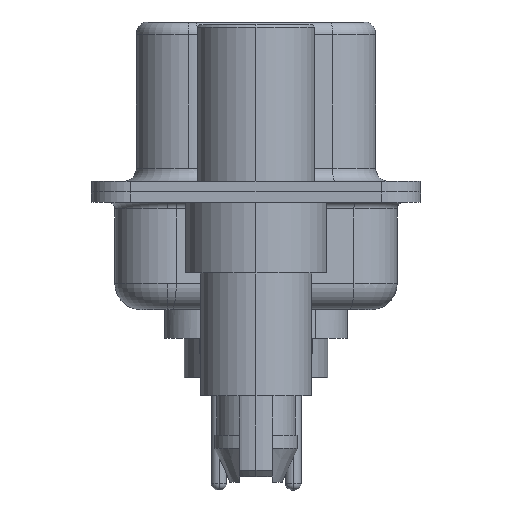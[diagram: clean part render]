
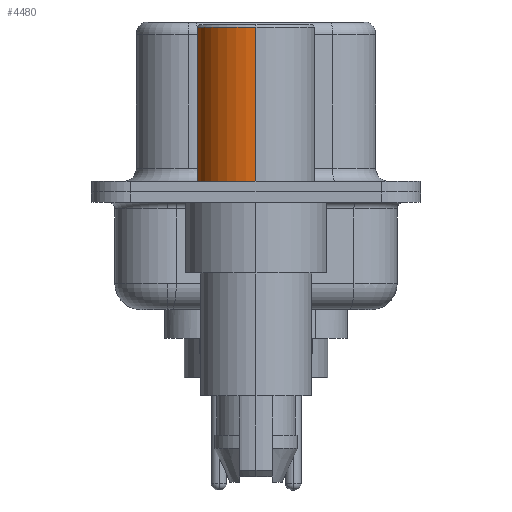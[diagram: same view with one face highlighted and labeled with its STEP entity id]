
A CAD part, left-side view. The second image highlights one B-rep face of the part: STEP entity #4480.
In plain terms, the highlighted cylindrical face has radius 2.25 mm (diameter 4.5 mm), a partial arc.
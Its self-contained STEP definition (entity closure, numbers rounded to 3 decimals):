
#163 = CIRCLE ( 'NONE', #2171, 2.25 ) ;
#1712 = CYLINDRICAL_SURFACE ( 'NONE', #19485, 2.25 ) ;
#1921 = CARTESIAN_POINT ( 'NONE',  ( 0., 0., 6.3 ) ) ;
#2171 = AXIS2_PLACEMENT_3D ( 'NONE', #12590, #12512, #12426 ) ;
#2316 = LINE ( 'NONE', #9059, #10362 ) ;
#3195 = CIRCLE ( 'NONE', #5423, 2.25 ) ;
#3201 = VERTEX_POINT ( 'NONE', #20568 ) ;
#3475 = ORIENTED_EDGE ( 'NONE', *, *, #18322, .F. ) ;
#3570 = DIRECTION ( 'NONE',  ( 1., 0., 0. ) ) ;
#3793 = EDGE_CURVE ( 'NONE', #5010, #3201, #163, .T. ) ;
#4480 = ADVANCED_FACE ( 'NONE', ( #14508 ), #1712, .T. ) ;
#5010 = VERTEX_POINT ( 'NONE', #9778 ) ;
#5423 = AXIS2_PLACEMENT_3D ( 'NONE', #1921, #13178, #3570 ) ;
#6766 = DIRECTION ( 'NONE',  ( 0., 0., 1. ) ) ;
#7247 = ORIENTED_EDGE ( 'NONE', *, *, #20223, .F. ) ;
#8501 = EDGE_CURVE ( 'NONE', #3201, #12145, #2316, .T. ) ;
#8787 = ORIENTED_EDGE ( 'NONE', *, *, #8501, .T. ) ;
#8957 = CARTESIAN_POINT ( 'NONE',  ( -2.25, 0., 6.3 ) ) ;
#9059 = CARTESIAN_POINT ( 'NONE',  ( -2.25, 0., 0.581 ) ) ;
#9778 = CARTESIAN_POINT ( 'NONE',  ( 2.25, 0., 0.4 ) ) ;
#9941 = CARTESIAN_POINT ( 'NONE',  ( 2.25, 0., 0.581 ) ) ;
#10362 = VECTOR ( 'NONE', #12227, 1000. ) ;
#10693 = CARTESIAN_POINT ( 'NONE',  ( 0., 0., 0.581 ) ) ;
#12145 = VERTEX_POINT ( 'NONE', #8957 ) ;
#12227 = DIRECTION ( 'NONE',  ( 0., 0., 1. ) ) ;
#12426 = DIRECTION ( 'NONE',  ( 1., 0., 0. ) ) ;
#12512 = DIRECTION ( 'NONE',  ( 0., 0., 1. ) ) ;
#12590 = CARTESIAN_POINT ( 'NONE',  ( 0., 0., 0.4 ) ) ;
#12926 = VECTOR ( 'NONE', #6766, 1000. ) ;
#13178 = DIRECTION ( 'NONE',  ( 0., 0., 1. ) ) ;
#13598 = DIRECTION ( 'NONE',  ( 0., 0., 1. ) ) ;
#13935 = VERTEX_POINT ( 'NONE', #15448 ) ;
#14115 = ORIENTED_EDGE ( 'NONE', *, *, #3793, .T. ) ;
#14300 = DIRECTION ( 'NONE',  ( 1., 0., 0. ) ) ;
#14508 = FACE_OUTER_BOUND ( 'NONE', #19264, .T. ) ;
#15448 = CARTESIAN_POINT ( 'NONE',  ( 2.25, 0., 6.3 ) ) ;
#17119 = LINE ( 'NONE', #9941, #12926 ) ;
#18322 = EDGE_CURVE ( 'NONE', #13935, #12145, #3195, .T. ) ;
#19264 = EDGE_LOOP ( 'NONE', ( #14115, #8787, #3475, #7247 ) ) ;
#19485 = AXIS2_PLACEMENT_3D ( 'NONE', #10693, #13598, #14300 ) ;
#20223 = EDGE_CURVE ( 'NONE', #5010, #13935, #17119, .T. ) ;
#20568 = CARTESIAN_POINT ( 'NONE',  ( -2.25, 0., 0.4 ) ) ;
